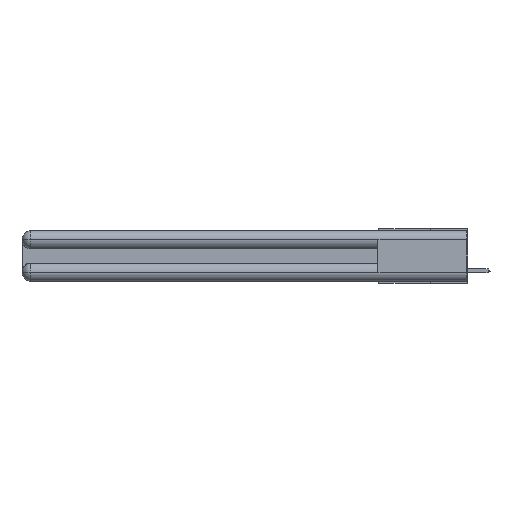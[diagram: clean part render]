
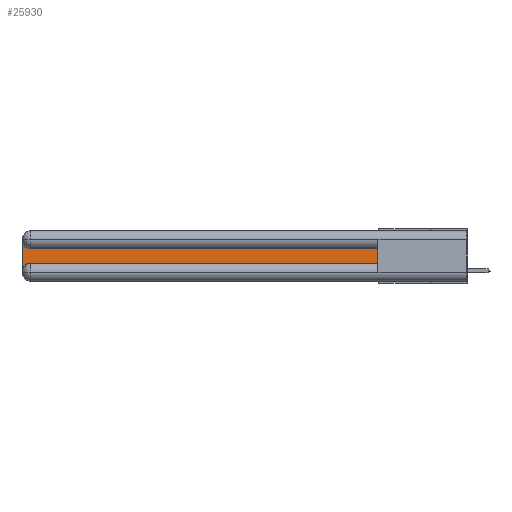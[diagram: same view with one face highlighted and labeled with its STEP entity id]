
A CAD part, left-side view. The second image highlights one B-rep face of the part: STEP entity #25930.
In plain terms, the highlighted planar face has unit normal (-1, 0, 0).
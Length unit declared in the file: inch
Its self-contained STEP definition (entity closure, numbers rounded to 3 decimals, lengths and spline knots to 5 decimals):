
#790 = VERTEX_POINT ( 'NONE', #25482 ) ;
#836 = DIRECTION ( 'NONE',  ( 1., 0., 0. ) ) ;
#1508 = AXIS2_PLACEMENT_3D ( 'NONE', #22689, #11454, #6844 ) ;
#1844 = CARTESIAN_POINT ( 'NONE',  ( 0.075, 2.94, -0.1225 ) ) ;
#2312 = AXIS2_PLACEMENT_3D ( 'NONE', #12221, #836, #14714 ) ;
#2553 = FACE_OUTER_BOUND ( 'NONE', #13428, .T. ) ;
#2973 = CARTESIAN_POINT ( 'NONE',  ( 0.075, 0.6, -0.1225 ) ) ;
#3826 = VERTEX_POINT ( 'NONE', #21320 ) ;
#4057 = EDGE_CURVE ( 'NONE', #24478, #790, #16313, .T. ) ;
#4339 = ORIENTED_EDGE ( 'NONE', *, *, #22425, .T. ) ;
#4447 = AXIS2_PLACEMENT_3D ( 'NONE', #12971, #19643, #10865 ) ;
#4881 = CARTESIAN_POINT ( 'NONE',  ( 0.075, 3., -0.2775 ) ) ;
#5039 = CARTESIAN_POINT ( 'NONE',  ( 0.075, 0.6, -0.2175 ) ) ;
#5112 = VECTOR ( 'NONE', #8003, 39.37008 ) ;
#5978 = ORIENTED_EDGE ( 'NONE', *, *, #4057, .T. ) ;
#6844 = DIRECTION ( 'NONE',  ( 0., 0., -1. ) ) ;
#7063 = VECTOR ( 'NONE', #11398, 39.37008 ) ;
#7107 = CARTESIAN_POINT ( 'NONE',  ( 0.075, 0.6, -0.1225 ) ) ;
#7792 = EDGE_CURVE ( 'NONE', #10440, #9537, #24535, .T. ) ;
#8003 = DIRECTION ( 'NONE',  ( 0., 0., 1. ) ) ;
#9283 = EDGE_CURVE ( 'NONE', #9537, #3826, #13326, .T. ) ;
#9537 = VERTEX_POINT ( 'NONE', #1844 ) ;
#9800 = ORIENTED_EDGE ( 'NONE', *, *, #13934, .T. ) ;
#10440 = VERTEX_POINT ( 'NONE', #2973 ) ;
#10865 = DIRECTION ( 'NONE',  ( 0., 0., -1. ) ) ;
#10969 = LINE ( 'NONE', #24784, #24153 ) ;
#11398 = DIRECTION ( 'NONE',  ( 0., 0., -1. ) ) ;
#11454 = DIRECTION ( 'NONE',  ( 1., 0., 0. ) ) ;
#12221 = CARTESIAN_POINT ( 'NONE',  ( 0.075, 3., -0.1225 ) ) ;
#12971 = CARTESIAN_POINT ( 'NONE',  ( 0.075, 2.94, -0.2775 ) ) ;
#13020 = LINE ( 'NONE', #28458, #5112 ) ;
#13326 = CIRCLE ( 'NONE', #1508, 0.06 ) ;
#13428 = EDGE_LOOP ( 'NONE', ( #18211, #20934, #4339, #5978, #9800, #25432 ) ) ;
#13934 = EDGE_CURVE ( 'NONE', #790, #15080, #10969, .T. ) ;
#14130 = DIRECTION ( 'NONE',  ( 0., 1., 0. ) ) ;
#14341 = EDGE_CURVE ( 'NONE', #15080, #10440, #13020, .T. ) ;
#14577 = VECTOR ( 'NONE', #14130, 39.37008 ) ;
#14714 = DIRECTION ( 'NONE',  ( 0., 0., -1. ) ) ;
#15080 = VERTEX_POINT ( 'NONE', #5039 ) ;
#16313 = CIRCLE ( 'NONE', #4447, 0.06 ) ;
#18211 = ORIENTED_EDGE ( 'NONE', *, *, #7792, .T. ) ;
#19096 = CARTESIAN_POINT ( 'NONE',  ( 0.075, 3., -0.2175 ) ) ;
#19643 = DIRECTION ( 'NONE',  ( 1., 0., 0. ) ) ;
#20934 = ORIENTED_EDGE ( 'NONE', *, *, #9283, .T. ) ;
#21320 = CARTESIAN_POINT ( 'NONE',  ( 0.075, 3., -0.0625 ) ) ;
#22425 = EDGE_CURVE ( 'NONE', #3826, #24478, #24225, .T. ) ;
#22689 = CARTESIAN_POINT ( 'NONE',  ( 0.075, 2.94, -0.0625 ) ) ;
#23979 = PLANE ( 'NONE',  #2312 ) ;
#24153 = VECTOR ( 'NONE', #27827, 39.37008 ) ;
#24225 = LINE ( 'NONE', #19096, #7063 ) ;
#24478 = VERTEX_POINT ( 'NONE', #4881 ) ;
#24535 = LINE ( 'NONE', #7107, #14577 ) ;
#24784 = CARTESIAN_POINT ( 'NONE',  ( 0.075, 0.6, -0.2175 ) ) ;
#25432 = ORIENTED_EDGE ( 'NONE', *, *, #14341, .T. ) ;
#25482 = CARTESIAN_POINT ( 'NONE',  ( 0.075, 2.94, -0.2175 ) ) ;
#25930 = ADVANCED_FACE ( 'NONE', ( #2553 ), #23979, .F. ) ;
#27827 = DIRECTION ( 'NONE',  ( 0., -1., 0. ) ) ;
#28458 = CARTESIAN_POINT ( 'NONE',  ( 0.075, 0.6, -0.2175 ) ) ;
